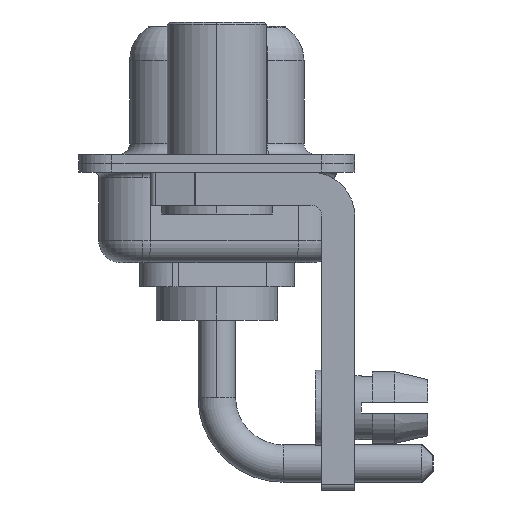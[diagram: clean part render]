
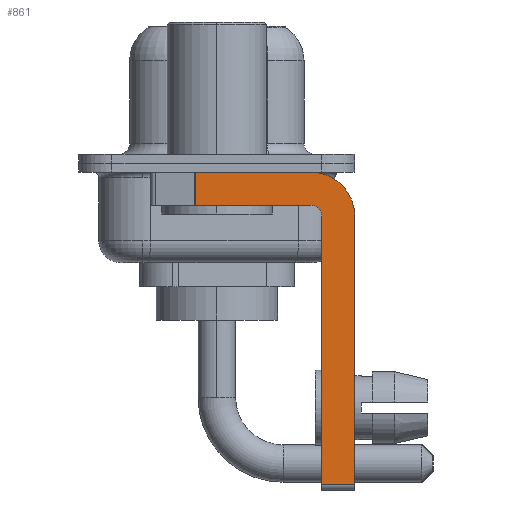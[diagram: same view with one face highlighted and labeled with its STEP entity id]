
A CAD part, left-side view. The second image highlights one B-rep face of the part: STEP entity #861.
In plain terms, the highlighted planar face has unit normal (-1, 0, 0).
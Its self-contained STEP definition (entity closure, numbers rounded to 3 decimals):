
#195 = VERTEX_POINT ( 'NONE', #10435 ) ;
#328 = CARTESIAN_POINT ( 'NONE',  ( -2.9, 0.978, -1.9 ) ) ;
#861 = ADVANCED_FACE ( 'NONE', ( #4410 ), #4229, .F. ) ;
#915 = CARTESIAN_POINT ( 'NONE',  ( -2.9, -4.25, -1.9 ) ) ;
#1689 = DIRECTION ( 'NONE',  ( 0., -1., 0. ) ) ;
#2230 = VECTOR ( 'NONE', #17144, 1000. ) ;
#2367 = CARTESIAN_POINT ( 'NONE',  ( -2.9, -4.25, -14.55 ) ) ;
#2878 = CARTESIAN_POINT ( 'NONE',  ( -2.9, -4.25, -2.4 ) ) ;
#3707 = LINE ( 'NONE', #8121, #15260 ) ;
#3771 = CARTESIAN_POINT ( 'NONE',  ( -2.9, 0.978, -1.9 ) ) ;
#3780 = DIRECTION ( 'NONE',  ( 0., 0., -1. ) ) ;
#4229 = PLANE ( 'NONE',  #11821 ) ;
#4323 = DIRECTION ( 'NONE',  ( 0., 0., -1. ) ) ;
#4410 = FACE_OUTER_BOUND ( 'NONE', #14982, .T. ) ;
#4513 = CARTESIAN_POINT ( 'NONE',  ( -2.9, 0.978, -0.4 ) ) ;
#4638 = LINE ( 'NONE', #11805, #2230 ) ;
#4731 = LINE ( 'NONE', #7696, #11496 ) ;
#4759 = VERTEX_POINT ( 'NONE', #13260 ) ;
#4767 = VERTEX_POINT ( 'NONE', #915 ) ;
#5383 = DIRECTION ( 'NONE',  ( 1., 0., 0. ) ) ;
#7100 = ORIENTED_EDGE ( 'NONE', *, *, #8256, .T. ) ;
#7108 = CARTESIAN_POINT ( 'NONE',  ( -2.9, 3., -0.4 ) ) ;
#7604 = ORIENTED_EDGE ( 'NONE', *, *, #17219, .F. ) ;
#7696 = CARTESIAN_POINT ( 'NONE',  ( -2.9, -4.75, -14.8 ) ) ;
#8121 = CARTESIAN_POINT ( 'NONE',  ( -2.9, -6.25, -2.4 ) ) ;
#8256 = EDGE_CURVE ( 'NONE', #14790, #17734, #14627, .T. ) ;
#8887 = ORIENTED_EDGE ( 'NONE', *, *, #17590, .F. ) ;
#8975 = CARTESIAN_POINT ( 'NONE',  ( -2.9, -4.25, -2.4 ) ) ;
#9148 = DIRECTION ( 'NONE',  ( 0., -1., 0. ) ) ;
#9847 = LINE ( 'NONE', #7108, #11015 ) ;
#10431 = DIRECTION ( 'NONE',  ( 0., 0., 1. ) ) ;
#10435 = CARTESIAN_POINT ( 'NONE',  ( -2.9, -4.25, -0.4 ) ) ;
#10436 = AXIS2_PLACEMENT_3D ( 'NONE', #10663, #5383, #3780 ) ;
#10604 = ORIENTED_EDGE ( 'NONE', *, *, #14333, .F. ) ;
#10663 = CARTESIAN_POINT ( 'NONE',  ( -2.9, -4.25, -2.4 ) ) ;
#10881 = ORIENTED_EDGE ( 'NONE', *, *, #12416, .F. ) ;
#11015 = VECTOR ( 'NONE', #1689, 1000. ) ;
#11044 = DIRECTION ( 'NONE',  ( 0., 0., -1. ) ) ;
#11172 = ORIENTED_EDGE ( 'NONE', *, *, #17197, .T. ) ;
#11485 = DIRECTION ( 'NONE',  ( 1., 0., 0. ) ) ;
#11496 = VECTOR ( 'NONE', #10431, 1000. ) ;
#11698 = VERTEX_POINT ( 'NONE', #13086 ) ;
#11805 = CARTESIAN_POINT ( 'NONE',  ( -2.9, -4.25, -1.9 ) ) ;
#11821 = AXIS2_PLACEMENT_3D ( 'NONE', #2878, #11485, #4323 ) ;
#12389 = CARTESIAN_POINT ( 'NONE',  ( -2.9, -6.25, -14.55 ) ) ;
#12416 = EDGE_CURVE ( 'NONE', #11698, #17734, #3707, .T. ) ;
#12515 = ORIENTED_EDGE ( 'NONE', *, *, #14331, .F. ) ;
#12879 = ORIENTED_EDGE ( 'NONE', *, *, #16374, .F. ) ;
#13086 = CARTESIAN_POINT ( 'NONE',  ( -2.9, -6.25, -2.4 ) ) ;
#13088 = DIRECTION ( 'NONE',  ( -1., 0., 0. ) ) ;
#13146 = VECTOR ( 'NONE', #9148, 1000. ) ;
#13260 = CARTESIAN_POINT ( 'NONE',  ( -2.9, -4.75, -2.4 ) ) ;
#13315 = AXIS2_PLACEMENT_3D ( 'NONE', #8975, #13088, #15709 ) ;
#14311 = CARTESIAN_POINT ( 'NONE',  ( -2.9, -4.75, -14.55 ) ) ;
#14331 = EDGE_CURVE ( 'NONE', #4767, #15399, #4638, .T. ) ;
#14333 = EDGE_CURVE ( 'NONE', #14790, #4759, #4731, .T. ) ;
#14491 = CIRCLE ( 'NONE', #10436, 2. ) ;
#14627 = LINE ( 'NONE', #2367, #13146 ) ;
#14790 = VERTEX_POINT ( 'NONE', #14311 ) ;
#14982 = EDGE_LOOP ( 'NONE', ( #7604, #11172, #12515, #12879, #10604, #7100, #10881, #8887 ) ) ;
#15260 = VECTOR ( 'NONE', #16301, 1000. ) ;
#15390 = LINE ( 'NONE', #328, #17093 ) ;
#15399 = VERTEX_POINT ( 'NONE', #3771 ) ;
#15709 = DIRECTION ( 'NONE',  ( 0., 0., 1. ) ) ;
#16200 = CIRCLE ( 'NONE', #13315, 0.5 ) ;
#16301 = DIRECTION ( 'NONE',  ( 0., 0., -1. ) ) ;
#16374 = EDGE_CURVE ( 'NONE', #4759, #4767, #16200, .T. ) ;
#16604 = VERTEX_POINT ( 'NONE', #4513 ) ;
#17093 = VECTOR ( 'NONE', #11044, 1000. ) ;
#17144 = DIRECTION ( 'NONE',  ( 0., 1., 0. ) ) ;
#17197 = EDGE_CURVE ( 'NONE', #16604, #15399, #15390, .T. ) ;
#17219 = EDGE_CURVE ( 'NONE', #16604, #195, #9847, .T. ) ;
#17590 = EDGE_CURVE ( 'NONE', #195, #11698, #14491, .T. ) ;
#17734 = VERTEX_POINT ( 'NONE', #12389 ) ;
